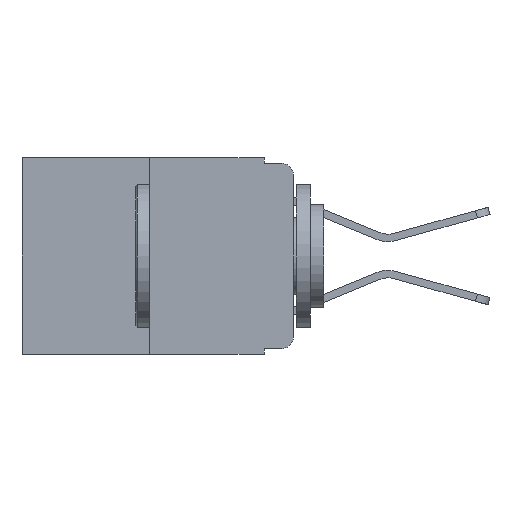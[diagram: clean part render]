
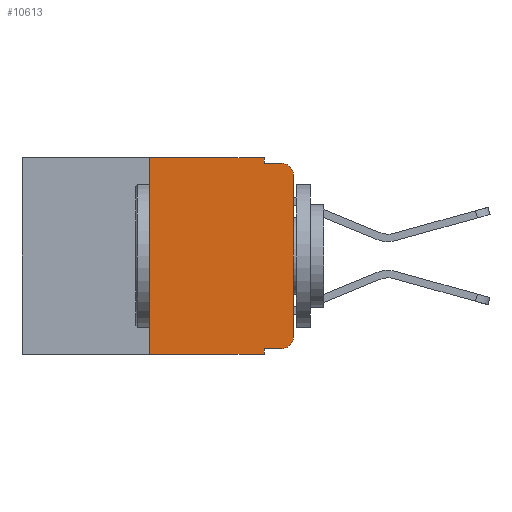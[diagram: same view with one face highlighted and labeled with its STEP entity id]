
A CAD part, left-side view. The second image highlights one B-rep face of the part: STEP entity #10613.
In plain terms, the highlighted planar face has unit normal (-1, 0, 0).
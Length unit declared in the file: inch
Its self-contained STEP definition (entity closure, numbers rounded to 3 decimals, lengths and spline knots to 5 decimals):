
#78 = ORIENTED_EDGE ( 'NONE', *, *, #279, .F. ) ;
#178 = VECTOR ( 'NONE', #13627, 39.37008 ) ;
#260 = DIRECTION ( 'NONE',  ( 0., -1., 0. ) ) ;
#279 = EDGE_CURVE ( 'NONE', #8279, #8482, #2070, .T. ) ;
#583 = VERTEX_POINT ( 'NONE', #9699 ) ;
#784 = DIRECTION ( 'NONE',  ( 0., -1., 0. ) ) ;
#833 = CARTESIAN_POINT ( 'NONE',  ( 0., 0.051, 0. ) ) ;
#1002 = ORIENTED_EDGE ( 'NONE', *, *, #7910, .F. ) ;
#1063 = CARTESIAN_POINT ( 'NONE',  ( 0., 0.25, -0.343 ) ) ;
#1130 = LINE ( 'NONE', #7465, #10688 ) ;
#1247 = ORIENTED_EDGE ( 'NONE', *, *, #11955, .T. ) ;
#1500 = CARTESIAN_POINT ( 'NONE',  ( 0., 0.051, -0.333 ) ) ;
#1552 = CARTESIAN_POINT ( 'NONE',  ( 0., 0.051, 0. ) ) ;
#1811 = ORIENTED_EDGE ( 'NONE', *, *, #4489, .F. ) ;
#1986 = CARTESIAN_POINT ( 'NONE',  ( 0., 0.02, -0.03 ) ) ;
#2070 = LINE ( 'NONE', #833, #8384 ) ;
#2290 = CIRCLE ( 'NONE', #10945, 0.02 ) ;
#2572 = ORIENTED_EDGE ( 'NONE', *, *, #11284, .F. ) ;
#2748 = VERTEX_POINT ( 'NONE', #1552 ) ;
#2764 = DIRECTION ( 'NONE',  ( -1., 0., 0. ) ) ;
#2795 = VECTOR ( 'NONE', #784, 39.37008 ) ;
#3035 = ORIENTED_EDGE ( 'NONE', *, *, #15327, .T. ) ;
#3098 = ORIENTED_EDGE ( 'NONE', *, *, #8755, .T. ) ;
#3194 = DIRECTION ( 'NONE',  ( 0., 0., -1. ) ) ;
#3213 = DIRECTION ( 'NONE',  ( 0., 0., -1. ) ) ;
#3491 = CARTESIAN_POINT ( 'NONE',  ( 0., 0.051, -0.343 ) ) ;
#3657 = EDGE_CURVE ( 'NONE', #13796, #11086, #3926, .T. ) ;
#3762 = VERTEX_POINT ( 'NONE', #7443 ) ;
#3926 = LINE ( 'NONE', #5833, #178 ) ;
#4035 = DIRECTION ( 'NONE',  ( 0., 0., -1. ) ) ;
#4242 = CARTESIAN_POINT ( 'NONE',  ( 0., 0.25, 0. ) ) ;
#4436 = VECTOR ( 'NONE', #260, 39.37008 ) ;
#4489 = EDGE_CURVE ( 'NONE', #2748, #11264, #7640, .T. ) ;
#4529 = CARTESIAN_POINT ( 'NONE',  ( 0., 0.473, 0. ) ) ;
#4619 = ORIENTED_EDGE ( 'NONE', *, *, #12240, .T. ) ;
#4797 = CARTESIAN_POINT ( 'NONE',  ( 0., 0.051, -0.01 ) ) ;
#5807 = DIRECTION ( 'NONE',  ( 0., 0., -1. ) ) ;
#5833 = CARTESIAN_POINT ( 'NONE',  ( 0., 0.25, 0. ) ) ;
#6022 = VERTEX_POINT ( 'NONE', #14659 ) ;
#6136 = LINE ( 'NONE', #11923, #2795 ) ;
#7152 = AXIS2_PLACEMENT_3D ( 'NONE', #4529, #13136, #5807 ) ;
#7247 = VECTOR ( 'NONE', #4035, 39.37008 ) ;
#7443 = CARTESIAN_POINT ( 'NONE',  ( 0., 0., -0.03 ) ) ;
#7465 = CARTESIAN_POINT ( 'NONE',  ( 0., 0.051, -0.01 ) ) ;
#7640 = LINE ( 'NONE', #8216, #7247 ) ;
#7827 = LINE ( 'NONE', #1500, #4436 ) ;
#7910 = EDGE_CURVE ( 'NONE', #11264, #12179, #1130, .T. ) ;
#8216 = CARTESIAN_POINT ( 'NONE',  ( 0., 0.051, 0. ) ) ;
#8279 = VERTEX_POINT ( 'NONE', #11899 ) ;
#8384 = VECTOR ( 'NONE', #3194, 39.37008 ) ;
#8482 = VERTEX_POINT ( 'NONE', #3491 ) ;
#8755 = EDGE_CURVE ( 'NONE', #3762, #12179, #2290, .T. ) ;
#8833 = LINE ( 'NONE', #13280, #14423 ) ;
#9211 = EDGE_LOOP ( 'NONE', ( #1247, #3098, #1002, #1811, #2572, #13656, #3035, #78, #4619, #14383 ) ) ;
#9699 = CARTESIAN_POINT ( 'NONE',  ( 0., 0., -0.313 ) ) ;
#9858 = FACE_OUTER_BOUND ( 'NONE', #9211, .T. ) ;
#9961 = DIRECTION ( 'NONE',  ( 0., -1., 0. ) ) ;
#10247 = CARTESIAN_POINT ( 'NONE',  ( 0., 0.02, -0.313 ) ) ;
#10412 = AXIS2_PLACEMENT_3D ( 'NONE', #10247, #2764, #11464 ) ;
#10613 = ADVANCED_FACE ( 'NONE', ( #9858 ), #11939, .F. ) ;
#10682 = DIRECTION ( 'NONE',  ( -1., 0., 0. ) ) ;
#10688 = VECTOR ( 'NONE', #9961, 39.37008 ) ;
#10945 = AXIS2_PLACEMENT_3D ( 'NONE', #1986, #10682, #3213 ) ;
#11086 = VERTEX_POINT ( 'NONE', #4242 ) ;
#11264 = VERTEX_POINT ( 'NONE', #4797 ) ;
#11284 = EDGE_CURVE ( 'NONE', #11086, #2748, #13207, .T. ) ;
#11464 = DIRECTION ( 'NONE',  ( 0., 0., -1. ) ) ;
#11472 = EDGE_CURVE ( 'NONE', #6022, #583, #15509, .T. ) ;
#11899 = CARTESIAN_POINT ( 'NONE',  ( 0., 0.051, -0.333 ) ) ;
#11923 = CARTESIAN_POINT ( 'NONE',  ( 0., 0.473, -0.343 ) ) ;
#11939 = PLANE ( 'NONE',  #7152 ) ;
#11955 = EDGE_CURVE ( 'NONE', #583, #3762, #8833, .T. ) ;
#12009 = DIRECTION ( 'NONE',  ( 0., 0., 1. ) ) ;
#12179 = VERTEX_POINT ( 'NONE', #12517 ) ;
#12226 = CARTESIAN_POINT ( 'NONE',  ( 0., 0.473, 0. ) ) ;
#12240 = EDGE_CURVE ( 'NONE', #8279, #6022, #7827, .T. ) ;
#12517 = CARTESIAN_POINT ( 'NONE',  ( 0., 0.02, -0.01 ) ) ;
#13136 = DIRECTION ( 'NONE',  ( 1., 0., 0. ) ) ;
#13207 = LINE ( 'NONE', #12226, #15909 ) ;
#13280 = CARTESIAN_POINT ( 'NONE',  ( 0., 0., 0. ) ) ;
#13454 = DIRECTION ( 'NONE',  ( 0., -1., 0. ) ) ;
#13627 = DIRECTION ( 'NONE',  ( 0., 0., 1. ) ) ;
#13656 = ORIENTED_EDGE ( 'NONE', *, *, #3657, .F. ) ;
#13796 = VERTEX_POINT ( 'NONE', #1063 ) ;
#14383 = ORIENTED_EDGE ( 'NONE', *, *, #11472, .T. ) ;
#14423 = VECTOR ( 'NONE', #12009, 39.37008 ) ;
#14659 = CARTESIAN_POINT ( 'NONE',  ( 0., 0.02, -0.333 ) ) ;
#15327 = EDGE_CURVE ( 'NONE', #13796, #8482, #6136, .T. ) ;
#15509 = CIRCLE ( 'NONE', #10412, 0.02 ) ;
#15909 = VECTOR ( 'NONE', #13454, 39.37008 ) ;
